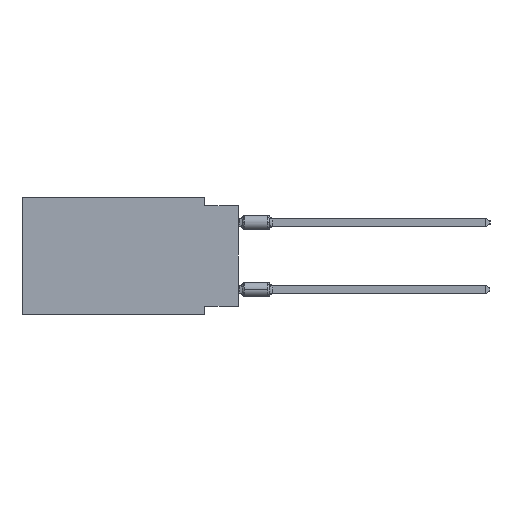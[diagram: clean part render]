
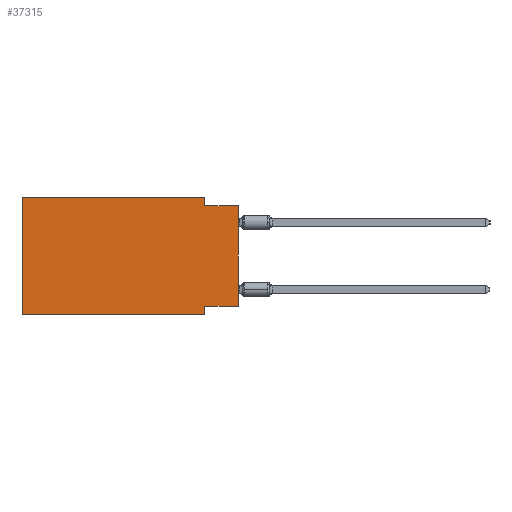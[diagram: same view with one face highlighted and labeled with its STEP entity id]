
A CAD part, left-side view. The second image highlights one B-rep face of the part: STEP entity #37315.
In plain terms, the highlighted planar face has unit normal (-1, 0, 0).
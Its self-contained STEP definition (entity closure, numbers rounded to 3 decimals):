
#3521 = DIRECTION ( 'NONE',  ( 0., -1., 0. ) ) ;
#3725 = CARTESIAN_POINT ( 'NONE',  ( 0., 2.54, -0.635 ) ) ;
#3936 = CARTESIAN_POINT ( 'NONE',  ( 0., 2.54, 0. ) ) ;
#4184 = ORIENTED_EDGE ( 'NONE', *, *, #59283, .F. ) ;
#4807 = CARTESIAN_POINT ( 'NONE',  ( 0., 16.383, 0. ) ) ;
#5663 = VECTOR ( 'NONE', #51535, 1000. ) ;
#5979 = CARTESIAN_POINT ( 'NONE',  ( 0., 2.54, -8.89 ) ) ;
#6873 = DIRECTION ( 'NONE',  ( 0., 0., 1. ) ) ;
#7281 = DIRECTION ( 'NONE',  ( 0., 1., 0. ) ) ;
#8516 = VERTEX_POINT ( 'NONE', #19397 ) ;
#8833 = VERTEX_POINT ( 'NONE', #43452 ) ;
#11461 = ORIENTED_EDGE ( 'NONE', *, *, #40329, .F. ) ;
#14378 = LINE ( 'NONE', #3936, #45217 ) ;
#14502 = LINE ( 'NONE', #34405, #31183 ) ;
#16702 = LINE ( 'NONE', #36577, #21054 ) ;
#17100 = VERTEX_POINT ( 'NONE', #41831 ) ;
#17628 = CARTESIAN_POINT ( 'NONE',  ( 0., 16.383, 0. ) ) ;
#18557 = LINE ( 'NONE', #53433, #23157 ) ;
#19286 = DIRECTION ( 'NONE',  ( 0., 0., -1. ) ) ;
#19397 = CARTESIAN_POINT ( 'NONE',  ( 0., 16.383, 0. ) ) ;
#20954 = DIRECTION ( 'NONE',  ( 0., -1., 0. ) ) ;
#21054 = VECTOR ( 'NONE', #6873, 1000. ) ;
#23157 = VECTOR ( 'NONE', #3521, 1000. ) ;
#24661 = VECTOR ( 'NONE', #20954, 1000. ) ;
#24729 = DIRECTION ( 'NONE',  ( 1., 0., 0. ) ) ;
#25860 = ORIENTED_EDGE ( 'NONE', *, *, #62793, .F. ) ;
#25900 = DIRECTION ( 'NONE',  ( 0., 0., -1. ) ) ;
#26468 = ORIENTED_EDGE ( 'NONE', *, *, #28160, .F. ) ;
#26522 = ORIENTED_EDGE ( 'NONE', *, *, #48817, .T. ) ;
#27556 = VERTEX_POINT ( 'NONE', #63264 ) ;
#28160 = EDGE_CURVE ( 'NONE', #17100, #42201, #56566, .T. ) ;
#28514 = ORIENTED_EDGE ( 'NONE', *, *, #56157, .F. ) ;
#28891 = DIRECTION ( 'NONE',  ( 0., -1., 0. ) ) ;
#29631 = FACE_OUTER_BOUND ( 'NONE', #55545, .T. ) ;
#31183 = VECTOR ( 'NONE', #28891, 1000. ) ;
#31659 = LINE ( 'NONE', #17628, #5663 ) ;
#31882 = ORIENTED_EDGE ( 'NONE', *, *, #54213, .F. ) ;
#33098 = ORIENTED_EDGE ( 'NONE', *, *, #62627, .T. ) ;
#34405 = CARTESIAN_POINT ( 'NONE',  ( 0., 16.383, -8.89 ) ) ;
#36577 = CARTESIAN_POINT ( 'NONE',  ( 0., 0., 0. ) ) ;
#37315 = ADVANCED_FACE ( 'NONE', ( #29631 ), #49495, .F. ) ;
#40329 = EDGE_CURVE ( 'NONE', #8516, #8833, #59797, .T. ) ;
#41831 = CARTESIAN_POINT ( 'NONE',  ( 0., 0., -8.255 ) ) ;
#42201 = VERTEX_POINT ( 'NONE', #43453 ) ;
#43452 = CARTESIAN_POINT ( 'NONE',  ( 0., 2.54, 0. ) ) ;
#43453 = CARTESIAN_POINT ( 'NONE',  ( 0., 2.54, -8.255 ) ) ;
#44350 = CARTESIAN_POINT ( 'NONE',  ( 0., 0., -0.635 ) ) ;
#45217 = VECTOR ( 'NONE', #19286, 1000. ) ;
#46350 = CARTESIAN_POINT ( 'NONE',  ( 0., 16.383, -8.89 ) ) ;
#47299 = VERTEX_POINT ( 'NONE', #44350 ) ;
#47831 = VECTOR ( 'NONE', #25900, 1000. ) ;
#48789 = VERTEX_POINT ( 'NONE', #46350 ) ;
#48817 = EDGE_CURVE ( 'NONE', #17100, #47299, #16702, .T. ) ;
#49495 = PLANE ( 'NONE',  #59740 ) ;
#50313 = CARTESIAN_POINT ( 'NONE',  ( 0., 16.383, 0. ) ) ;
#50887 = VERTEX_POINT ( 'NONE', #3725 ) ;
#51342 = CARTESIAN_POINT ( 'NONE',  ( 0., 0., -8.255 ) ) ;
#51535 = DIRECTION ( 'NONE',  ( 0., 0., 1. ) ) ;
#53433 = CARTESIAN_POINT ( 'NONE',  ( 0., 0., -0.635 ) ) ;
#54213 = EDGE_CURVE ( 'NONE', #50887, #47299, #18557, .T. ) ;
#55545 = EDGE_LOOP ( 'NONE', ( #26522, #31882, #28514, #11461, #4184, #33098, #25860, #26468 ) ) ;
#55898 = LINE ( 'NONE', #5979, #47831 ) ;
#56157 = EDGE_CURVE ( 'NONE', #8833, #50887, #14378, .T. ) ;
#56566 = LINE ( 'NONE', #51342, #56820 ) ;
#56820 = VECTOR ( 'NONE', #7281, 1000. ) ;
#59283 = EDGE_CURVE ( 'NONE', #48789, #8516, #31659, .T. ) ;
#59740 = AXIS2_PLACEMENT_3D ( 'NONE', #4807, #24729, #62117 ) ;
#59797 = LINE ( 'NONE', #50313, #24661 ) ;
#62117 = DIRECTION ( 'NONE',  ( 0., 0., -1. ) ) ;
#62627 = EDGE_CURVE ( 'NONE', #48789, #27556, #14502, .T. ) ;
#62793 = EDGE_CURVE ( 'NONE', #42201, #27556, #55898, .T. ) ;
#63264 = CARTESIAN_POINT ( 'NONE',  ( 0., 2.54, -8.89 ) ) ;
